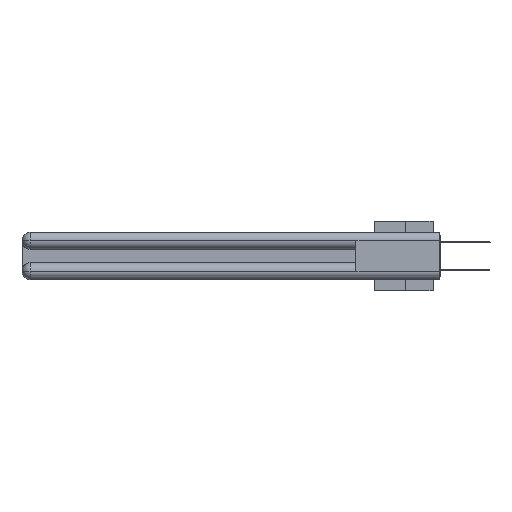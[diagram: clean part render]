
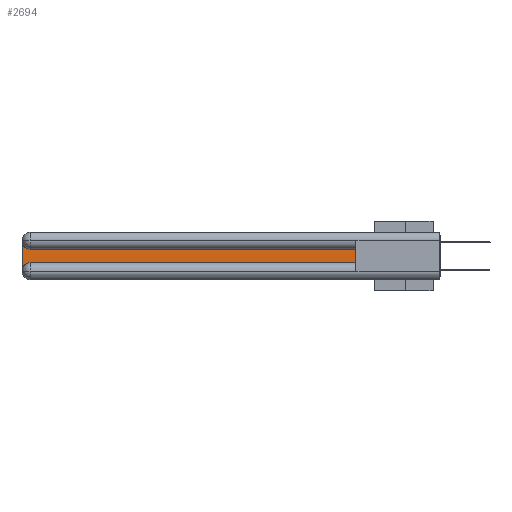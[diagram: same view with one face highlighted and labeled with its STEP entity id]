
A CAD part, left-side view. The second image highlights one B-rep face of the part: STEP entity #2694.
In plain terms, the highlighted planar face has unit normal (-1, 0, 0).
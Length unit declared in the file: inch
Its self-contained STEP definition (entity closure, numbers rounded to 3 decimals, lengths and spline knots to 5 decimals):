
#178 = CARTESIAN_POINT ( 'NONE',  ( 0.075, 2.94, -0.0625 ) ) ;
#1716 = DIRECTION ( 'NONE',  ( 0., 0., 1. ) ) ;
#2167 = VECTOR ( 'NONE', #1716, 39.37008 ) ;
#2375 = CIRCLE ( 'NONE', #24580, 0.06 ) ;
#2694 = ADVANCED_FACE ( 'NONE', ( #4192 ), #29011, .F. ) ;
#2874 = DIRECTION ( 'NONE',  ( 0., 0., -1. ) ) ;
#2926 = LINE ( 'NONE', #4595, #33883 ) ;
#3074 = EDGE_CURVE ( 'NONE', #32078, #34635, #31259, .T. ) ;
#3210 = CARTESIAN_POINT ( 'NONE',  ( 0.075, 2.94, -0.1225 ) ) ;
#3341 = LINE ( 'NONE', #21987, #12935 ) ;
#3610 = EDGE_CURVE ( 'NONE', #3720, #25639, #2375, .T. ) ;
#3720 = VERTEX_POINT ( 'NONE', #3210 ) ;
#4192 = FACE_OUTER_BOUND ( 'NONE', #21226, .T. ) ;
#4595 = CARTESIAN_POINT ( 'NONE',  ( 0.075, 0.6, -0.2175 ) ) ;
#4948 = DIRECTION ( 'NONE',  ( 0., 1., 0. ) ) ;
#6527 = ORIENTED_EDGE ( 'NONE', *, *, #3610, .T. ) ;
#6863 = CARTESIAN_POINT ( 'NONE',  ( 0.075, 0.6, -0.2175 ) ) ;
#11259 = DIRECTION ( 'NONE',  ( 0., 0., -1. ) ) ;
#12297 = DIRECTION ( 'NONE',  ( 0., 0., -1. ) ) ;
#12417 = LINE ( 'NONE', #33343, #34686 ) ;
#12430 = DIRECTION ( 'NONE',  ( 1., 0., 0. ) ) ;
#12935 = VECTOR ( 'NONE', #4948, 39.37008 ) ;
#13609 = CARTESIAN_POINT ( 'NONE',  ( 0.075, 2.94, -0.2175 ) ) ;
#13939 = LINE ( 'NONE', #6863, #2167 ) ;
#14130 = DIRECTION ( 'NONE',  ( 1., 0., 0. ) ) ;
#15801 = ORIENTED_EDGE ( 'NONE', *, *, #24290, .T. ) ;
#16302 = VERTEX_POINT ( 'NONE', #32589 ) ;
#17061 = CARTESIAN_POINT ( 'NONE',  ( 0.075, 0.6, -0.2175 ) ) ;
#18336 = DIRECTION ( 'NONE',  ( 0., -1., 0. ) ) ;
#19484 = CARTESIAN_POINT ( 'NONE',  ( 0.075, 2.94, -0.2775 ) ) ;
#21226 = EDGE_LOOP ( 'NONE', ( #28757, #6527, #31564, #32963, #15801, #22669 ) ) ;
#21987 = CARTESIAN_POINT ( 'NONE',  ( 0.075, 0.6, -0.1225 ) ) ;
#22669 = ORIENTED_EDGE ( 'NONE', *, *, #30785, .T. ) ;
#23415 = AXIS2_PLACEMENT_3D ( 'NONE', #19484, #14130, #28477 ) ;
#24290 = EDGE_CURVE ( 'NONE', #34635, #26285, #2926, .T. ) ;
#24580 = AXIS2_PLACEMENT_3D ( 'NONE', #178, #31042, #2874 ) ;
#25639 = VERTEX_POINT ( 'NONE', #30659 ) ;
#26285 = VERTEX_POINT ( 'NONE', #17061 ) ;
#26318 = CARTESIAN_POINT ( 'NONE',  ( 0.075, 3., -0.1225 ) ) ;
#27372 = AXIS2_PLACEMENT_3D ( 'NONE', #26318, #12430, #12297 ) ;
#28477 = DIRECTION ( 'NONE',  ( 0., 0., -1. ) ) ;
#28757 = ORIENTED_EDGE ( 'NONE', *, *, #32196, .T. ) ;
#29011 = PLANE ( 'NONE',  #27372 ) ;
#29823 = CARTESIAN_POINT ( 'NONE',  ( 0.075, 3., -0.2775 ) ) ;
#30659 = CARTESIAN_POINT ( 'NONE',  ( 0.075, 3., -0.0625 ) ) ;
#30785 = EDGE_CURVE ( 'NONE', #26285, #16302, #13939, .T. ) ;
#31042 = DIRECTION ( 'NONE',  ( 1., 0., 0. ) ) ;
#31259 = CIRCLE ( 'NONE', #23415, 0.06 ) ;
#31564 = ORIENTED_EDGE ( 'NONE', *, *, #35427, .T. ) ;
#32078 = VERTEX_POINT ( 'NONE', #29823 ) ;
#32196 = EDGE_CURVE ( 'NONE', #16302, #3720, #3341, .T. ) ;
#32589 = CARTESIAN_POINT ( 'NONE',  ( 0.075, 0.6, -0.1225 ) ) ;
#32963 = ORIENTED_EDGE ( 'NONE', *, *, #3074, .T. ) ;
#33343 = CARTESIAN_POINT ( 'NONE',  ( 0.075, 3., -0.2175 ) ) ;
#33883 = VECTOR ( 'NONE', #18336, 39.37008 ) ;
#34635 = VERTEX_POINT ( 'NONE', #13609 ) ;
#34686 = VECTOR ( 'NONE', #11259, 39.37008 ) ;
#35427 = EDGE_CURVE ( 'NONE', #25639, #32078, #12417, .T. ) ;
